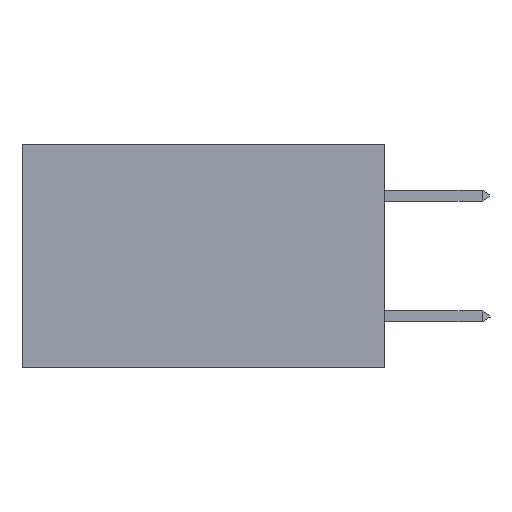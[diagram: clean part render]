
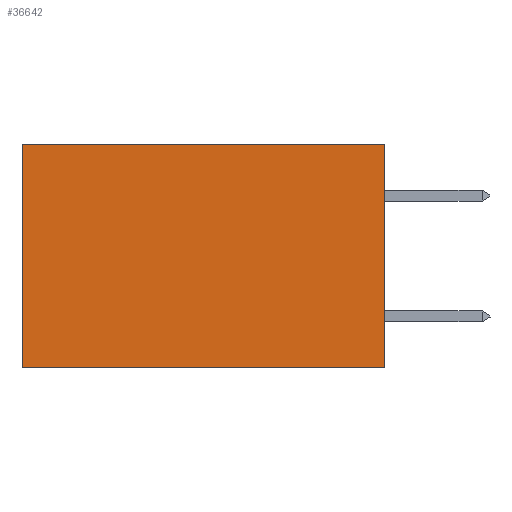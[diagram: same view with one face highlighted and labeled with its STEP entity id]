
A CAD part, left-side view. The second image highlights one B-rep face of the part: STEP entity #36642.
In plain terms, the highlighted planar face has unit normal (-1, 0, 0).
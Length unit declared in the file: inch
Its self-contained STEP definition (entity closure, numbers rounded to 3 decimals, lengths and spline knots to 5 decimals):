
#313 = VECTOR ( 'NONE', #11395, 39.37008 ) ;
#1029 = CARTESIAN_POINT ( 'NONE',  ( 0.2875, 0.6, -0.37 ) ) ;
#1358 = VERTEX_POINT ( 'NONE', #1029 ) ;
#2027 = VECTOR ( 'NONE', #35122, 39.37008 ) ;
#2400 = ORIENTED_EDGE ( 'NONE', *, *, #38897, .F. ) ;
#4379 = CARTESIAN_POINT ( 'NONE',  ( 0.2875, 0., 0. ) ) ;
#5473 = VECTOR ( 'NONE', #17880, 39.37008 ) ;
#6777 = VERTEX_POINT ( 'NONE', #15315 ) ;
#8228 = CARTESIAN_POINT ( 'NONE',  ( 0.2875, 0.6, 0. ) ) ;
#8727 = ORIENTED_EDGE ( 'NONE', *, *, #32727, .T. ) ;
#10810 = CARTESIAN_POINT ( 'NONE',  ( 0.2875, 0., -0.37 ) ) ;
#11395 = DIRECTION ( 'NONE',  ( 0., 0., -1. ) ) ;
#11486 = AXIS2_PLACEMENT_3D ( 'NONE', #12341, #34360, #15523 ) ;
#11545 = CARTESIAN_POINT ( 'NONE',  ( 0.2875, 0., 0. ) ) ;
#12108 = ORIENTED_EDGE ( 'NONE', *, *, #22836, .T. ) ;
#12341 = CARTESIAN_POINT ( 'NONE',  ( 0.2875, 0., 0. ) ) ;
#12433 = ORIENTED_EDGE ( 'NONE', *, *, #39778, .F. ) ;
#15315 = CARTESIAN_POINT ( 'NONE',  ( 0.2875, 0., 0. ) ) ;
#15523 = DIRECTION ( 'NONE',  ( 0., 0., -1. ) ) ;
#17880 = DIRECTION ( 'NONE',  ( 0., 0., -1. ) ) ;
#18494 = VERTEX_POINT ( 'NONE', #10810 ) ;
#18687 = LINE ( 'NONE', #25795, #2027 ) ;
#20349 = FACE_OUTER_BOUND ( 'NONE', #27484, .T. ) ;
#22208 = LINE ( 'NONE', #11545, #5473 ) ;
#22836 = EDGE_CURVE ( 'NONE', #6777, #23607, #39550, .T. ) ;
#23607 = VERTEX_POINT ( 'NONE', #27152 ) ;
#25795 = CARTESIAN_POINT ( 'NONE',  ( 0.2875, 0., -0.37 ) ) ;
#27152 = CARTESIAN_POINT ( 'NONE',  ( 0.2875, 0.6, 0. ) ) ;
#27484 = EDGE_LOOP ( 'NONE', ( #8727, #2400, #12433, #12108 ) ) ;
#31167 = VECTOR ( 'NONE', #39047, 39.37008 ) ;
#31210 = PLANE ( 'NONE',  #11486 ) ;
#32727 = EDGE_CURVE ( 'NONE', #23607, #1358, #34647, .T. ) ;
#34360 = DIRECTION ( 'NONE',  ( 1., 0., 0. ) ) ;
#34647 = LINE ( 'NONE', #8228, #313 ) ;
#35122 = DIRECTION ( 'NONE',  ( 0., 1., 0. ) ) ;
#36642 = ADVANCED_FACE ( 'NONE', ( #20349 ), #31210, .F. ) ;
#38897 = EDGE_CURVE ( 'NONE', #18494, #1358, #18687, .T. ) ;
#39047 = DIRECTION ( 'NONE',  ( 0., 1., 0. ) ) ;
#39550 = LINE ( 'NONE', #4379, #31167 ) ;
#39778 = EDGE_CURVE ( 'NONE', #6777, #18494, #22208, .T. ) ;
